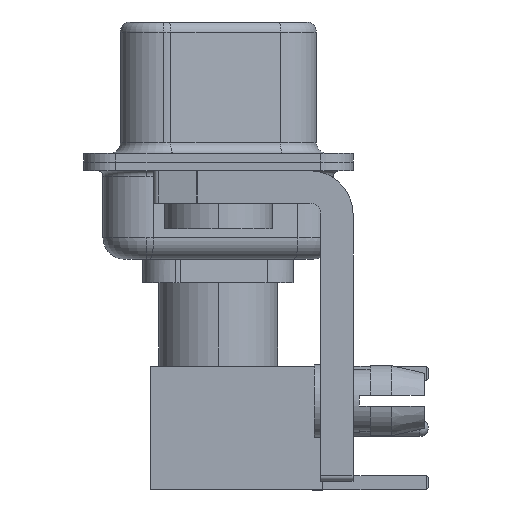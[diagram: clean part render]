
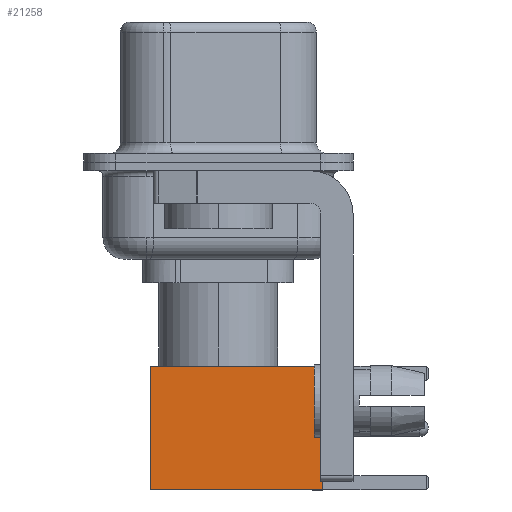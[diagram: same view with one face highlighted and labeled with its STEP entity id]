
A CAD part, left-side view. The second image highlights one B-rep face of the part: STEP entity #21258.
In plain terms, the highlighted face is planar.
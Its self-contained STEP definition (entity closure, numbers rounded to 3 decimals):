
#333 = ORIENTED_EDGE ( 'NONE', *, *, #15270, .T. ) ;
#445 = VERTEX_POINT ( 'NONE', #8987 ) ;
#1006 = LINE ( 'NONE', #21562, #13776 ) ;
#1177 = ORIENTED_EDGE ( 'NONE', *, *, #16573, .T. ) ;
#5161 = VERTEX_POINT ( 'NONE', #21537 ) ;
#5568 = ORIENTED_EDGE ( 'NONE', *, *, #16831, .F. ) ;
#6015 = CARTESIAN_POINT ( 'NONE',  ( 2.875, 2.875, 0. ) ) ;
#6307 = DIRECTION ( 'NONE',  ( -1., 0., 0. ) ) ;
#6711 = VECTOR ( 'NONE', #6307, 1000. ) ;
#8208 = EDGE_LOOP ( 'NONE', ( #1177, #333, #5568, #11164 ) ) ;
#8438 = CARTESIAN_POINT ( 'NONE',  ( 2.875, 2.875, 8. ) ) ;
#8609 = LINE ( 'NONE', #15458, #21745 ) ;
#8987 = CARTESIAN_POINT ( 'NONE',  ( -2.875, 2.875, 0. ) ) ;
#9383 = FACE_OUTER_BOUND ( 'NONE', #8208, .T. ) ;
#9558 = LINE ( 'NONE', #16404, #6711 ) ;
#10182 = DIRECTION ( 'NONE',  ( 0., 0., -1. ) ) ;
#10895 = VERTEX_POINT ( 'NONE', #19668 ) ;
#11100 = LINE ( 'NONE', #12993, #16330 ) ;
#11164 = ORIENTED_EDGE ( 'NONE', *, *, #19845, .F. ) ;
#11202 = DIRECTION ( 'NONE',  ( 0., 0., -1. ) ) ;
#12987 = DIRECTION ( 'NONE',  ( -1., 0., 0. ) ) ;
#12993 = CARTESIAN_POINT ( 'NONE',  ( 2.875, 2.875, 0. ) ) ;
#13060 = PLANE ( 'NONE',  #18969 ) ;
#13776 = VECTOR ( 'NONE', #12987, 1000. ) ;
#15270 = EDGE_CURVE ( 'NONE', #5161, #445, #1006, .T. ) ;
#15458 = CARTESIAN_POINT ( 'NONE',  ( -2.875, 2.875, 0. ) ) ;
#16225 = DIRECTION ( 'NONE',  ( 0., 1., 0. ) ) ;
#16330 = VECTOR ( 'NONE', #11202, 1000. ) ;
#16404 = CARTESIAN_POINT ( 'NONE',  ( 0., 2.875, 8. ) ) ;
#16573 = EDGE_CURVE ( 'NONE', #17982, #5161, #11100, .T. ) ;
#16831 = EDGE_CURVE ( 'NONE', #10895, #445, #8609, .T. ) ;
#17982 = VERTEX_POINT ( 'NONE', #8438 ) ;
#18969 = AXIS2_PLACEMENT_3D ( 'NONE', #6015, #16225, #19734 ) ;
#19668 = CARTESIAN_POINT ( 'NONE',  ( -2.875, 2.875, 8. ) ) ;
#19734 = DIRECTION ( 'NONE',  ( 0., 0., 1. ) ) ;
#19845 = EDGE_CURVE ( 'NONE', #17982, #10895, #9558, .T. ) ;
#21258 = ADVANCED_FACE ( 'NONE', ( #9383 ), #13060, .T. ) ;
#21537 = CARTESIAN_POINT ( 'NONE',  ( 2.875, 2.875, 0. ) ) ;
#21562 = CARTESIAN_POINT ( 'NONE',  ( 0., 2.875, 0. ) ) ;
#21745 = VECTOR ( 'NONE', #10182, 1000. ) ;
